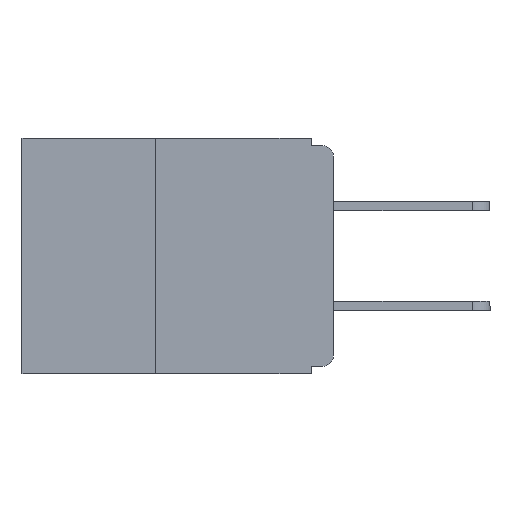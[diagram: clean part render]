
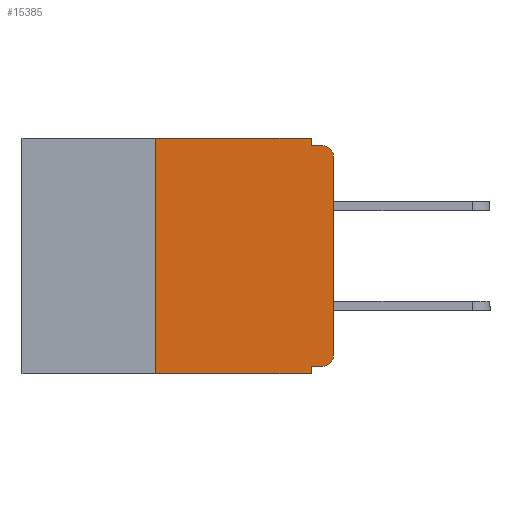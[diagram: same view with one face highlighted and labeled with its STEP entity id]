
A CAD part, left-side view. The second image highlights one B-rep face of the part: STEP entity #15385.
In plain terms, the highlighted planar face has unit normal (-1, 0, 0).
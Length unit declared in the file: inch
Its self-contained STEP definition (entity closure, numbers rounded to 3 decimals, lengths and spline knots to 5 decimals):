
#35 = VERTEX_POINT ( 'NONE', #18000 ) ;
#675 = EDGE_CURVE ( 'NONE', #12182, #5139, #27534, .T. ) ;
#1162 = CARTESIAN_POINT ( 'NONE',  ( 0., 0.031, -0.32 ) ) ;
#1327 = DIRECTION ( 'NONE',  ( 0., 0., -1. ) ) ;
#1389 = ORIENTED_EDGE ( 'NONE', *, *, #19522, .T. ) ;
#3258 = CARTESIAN_POINT ( 'NONE',  ( 0., 0., -0.32 ) ) ;
#3320 = LINE ( 'NONE', #24561, #26991 ) ;
#3547 = EDGE_CURVE ( 'NONE', #24080, #8238, #18673, .T. ) ;
#3578 = CARTESIAN_POINT ( 'NONE',  ( 0., 0.031, -0.33 ) ) ;
#4417 = ORIENTED_EDGE ( 'NONE', *, *, #675, .F. ) ;
#4849 = LINE ( 'NONE', #12619, #16387 ) ;
#5139 = VERTEX_POINT ( 'NONE', #11895 ) ;
#5334 = ORIENTED_EDGE ( 'NONE', *, *, #20939, .T. ) ;
#5878 = CARTESIAN_POINT ( 'NONE',  ( 0., 0., -0.025 ) ) ;
#6169 = VECTOR ( 'NONE', #11905, 39.37008 ) ;
#6183 = AXIS2_PLACEMENT_3D ( 'NONE', #10176, #27192, #12645 ) ;
#6547 = EDGE_CURVE ( 'NONE', #35, #12182, #4849, .T. ) ;
#6947 = LINE ( 'NONE', #28859, #6169 ) ;
#7036 = ORIENTED_EDGE ( 'NONE', *, *, #6547, .F. ) ;
#7094 = EDGE_CURVE ( 'NONE', #5139, #21595, #3320, .T. ) ;
#8238 = VERTEX_POINT ( 'NONE', #3578 ) ;
#10176 = CARTESIAN_POINT ( 'NONE',  ( 0., 0.015, -0.025 ) ) ;
#10571 = VERTEX_POINT ( 'NONE', #13220 ) ;
#10711 = CARTESIAN_POINT ( 'NONE',  ( 0., 0.015, -0.305 ) ) ;
#10971 = CARTESIAN_POINT ( 'NONE',  ( 0., 0.25, 0. ) ) ;
#11180 = CARTESIAN_POINT ( 'NONE',  ( 0., 0., -0.305 ) ) ;
#11855 = CARTESIAN_POINT ( 'NONE',  ( 0., 0., 0. ) ) ;
#11895 = CARTESIAN_POINT ( 'NONE',  ( 0., 0.031, 0. ) ) ;
#11905 = DIRECTION ( 'NONE',  ( 0., -1., 0. ) ) ;
#12182 = VERTEX_POINT ( 'NONE', #10971 ) ;
#12228 = VERTEX_POINT ( 'NONE', #11180 ) ;
#12454 = CIRCLE ( 'NONE', #6183, 0.015 ) ;
#12562 = DIRECTION ( 'NONE',  ( 0., 0., 1. ) ) ;
#12619 = CARTESIAN_POINT ( 'NONE',  ( 0., 0.25, -0.33 ) ) ;
#12645 = DIRECTION ( 'NONE',  ( 0., 0., -1. ) ) ;
#12723 = EDGE_CURVE ( 'NONE', #21087, #12228, #21753, .T. ) ;
#13150 = DIRECTION ( 'NONE',  ( 0., 0., -1. ) ) ;
#13220 = CARTESIAN_POINT ( 'NONE',  ( 0., 0.015, -0.01 ) ) ;
#14116 = CARTESIAN_POINT ( 'NONE',  ( 0., 0.437, 0. ) ) ;
#14312 = CARTESIAN_POINT ( 'NONE',  ( 0., 0.437, 0. ) ) ;
#15149 = VERTEX_POINT ( 'NONE', #5878 ) ;
#15385 = ADVANCED_FACE ( 'NONE', ( #19995 ), #26270, .F. ) ;
#16330 = CARTESIAN_POINT ( 'NONE',  ( 0., 0.437, -0.33 ) ) ;
#16387 = VECTOR ( 'NONE', #12562, 39.37008 ) ;
#16432 = DIRECTION ( 'NONE',  ( 0., -1., 0. ) ) ;
#16606 = DIRECTION ( 'NONE',  ( 0., 0., -1. ) ) ;
#18000 = CARTESIAN_POINT ( 'NONE',  ( 0., 0.25, -0.33 ) ) ;
#18517 = CARTESIAN_POINT ( 'NONE',  ( 0., 0.031, -0.33 ) ) ;
#18673 = LINE ( 'NONE', #18517, #30786 ) ;
#19522 = EDGE_CURVE ( 'NONE', #12228, #15149, #29997, .T. ) ;
#19589 = ORIENTED_EDGE ( 'NONE', *, *, #29647, .F. ) ;
#19995 = FACE_OUTER_BOUND ( 'NONE', #20931, .T. ) ;
#20538 = ORIENTED_EDGE ( 'NONE', *, *, #22238, .F. ) ;
#20931 = EDGE_LOOP ( 'NONE', ( #1389, #28750, #20538, #21334, #4417, #7036, #5334, #22631, #19589, #26411 ) ) ;
#20939 = EDGE_CURVE ( 'NONE', #35, #8238, #30644, .T. ) ;
#21087 = VERTEX_POINT ( 'NONE', #24190 ) ;
#21334 = ORIENTED_EDGE ( 'NONE', *, *, #7094, .F. ) ;
#21595 = VERTEX_POINT ( 'NONE', #30796 ) ;
#21753 = CIRCLE ( 'NONE', #27846, 0.015 ) ;
#21891 = VECTOR ( 'NONE', #26593, 39.37008 ) ;
#22238 = EDGE_CURVE ( 'NONE', #21595, #10571, #6947, .T. ) ;
#22631 = ORIENTED_EDGE ( 'NONE', *, *, #3547, .F. ) ;
#24080 = VERTEX_POINT ( 'NONE', #1162 ) ;
#24190 = CARTESIAN_POINT ( 'NONE',  ( 0., 0.015, -0.32 ) ) ;
#24561 = CARTESIAN_POINT ( 'NONE',  ( 0., 0.031, 0. ) ) ;
#25231 = DIRECTION ( 'NONE',  ( 0., 1., 0. ) ) ;
#26270 = PLANE ( 'NONE',  #27292 ) ;
#26392 = DIRECTION ( 'NONE',  ( 0., 0., 1. ) ) ;
#26411 = ORIENTED_EDGE ( 'NONE', *, *, #12723, .T. ) ;
#26593 = DIRECTION ( 'NONE',  ( 0., -1., 0. ) ) ;
#26848 = VECTOR ( 'NONE', #25231, 39.37008 ) ;
#26991 = VECTOR ( 'NONE', #30201, 39.37008 ) ;
#27192 = DIRECTION ( 'NONE',  ( -1., 0., 0. ) ) ;
#27292 = AXIS2_PLACEMENT_3D ( 'NONE', #14116, #31087, #16606 ) ;
#27534 = LINE ( 'NONE', #14312, #21891 ) ;
#27697 = DIRECTION ( 'NONE',  ( -1., 0., 0. ) ) ;
#27846 = AXIS2_PLACEMENT_3D ( 'NONE', #10711, #27697, #13150 ) ;
#28750 = ORIENTED_EDGE ( 'NONE', *, *, #28874, .T. ) ;
#28859 = CARTESIAN_POINT ( 'NONE',  ( 0., 0., -0.01 ) ) ;
#28874 = EDGE_CURVE ( 'NONE', #15149, #10571, #12454, .T. ) ;
#29097 = LINE ( 'NONE', #3258, #26848 ) ;
#29647 = EDGE_CURVE ( 'NONE', #21087, #24080, #29097, .T. ) ;
#29863 = VECTOR ( 'NONE', #16432, 39.37008 ) ;
#29997 = LINE ( 'NONE', #11855, #30763 ) ;
#30201 = DIRECTION ( 'NONE',  ( 0., 0., -1. ) ) ;
#30644 = LINE ( 'NONE', #16330, #29863 ) ;
#30763 = VECTOR ( 'NONE', #26392, 39.37008 ) ;
#30786 = VECTOR ( 'NONE', #1327, 39.37008 ) ;
#30796 = CARTESIAN_POINT ( 'NONE',  ( 0., 0.031, -0.01 ) ) ;
#31087 = DIRECTION ( 'NONE',  ( 1., 0., 0. ) ) ;
